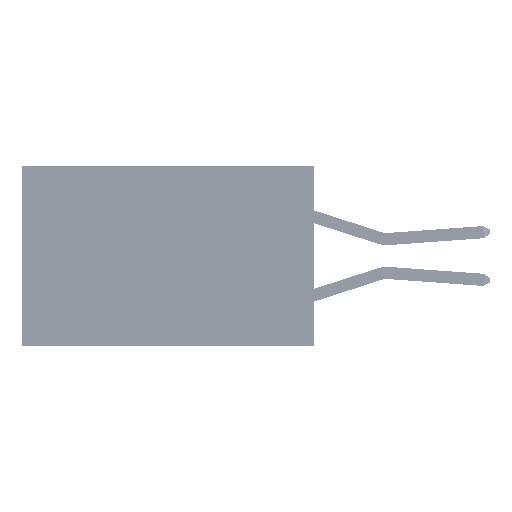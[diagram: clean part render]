
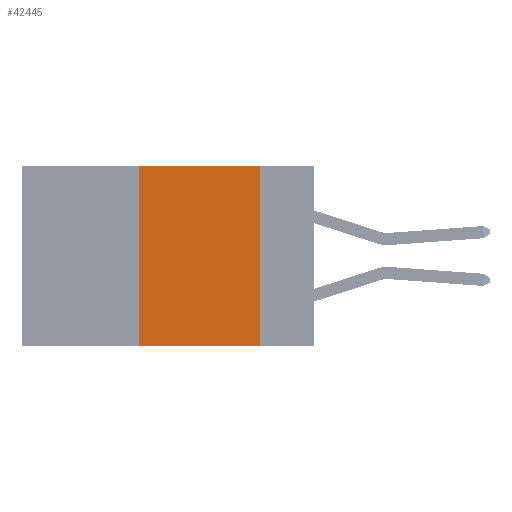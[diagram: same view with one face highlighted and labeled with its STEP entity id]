
A CAD part, left-side view. The second image highlights one B-rep face of the part: STEP entity #42445.
In plain terms, the highlighted planar face has unit normal (-1, 0, 0).
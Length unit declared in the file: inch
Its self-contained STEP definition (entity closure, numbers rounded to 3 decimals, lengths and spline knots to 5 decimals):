
#1733 = PLANE ( 'NONE',  #35816 ) ;
#5433 = EDGE_CURVE ( 'NONE', #27757, #46484, #41402, .T. ) ;
#5661 = DIRECTION ( 'NONE',  ( 1., 0., 0. ) ) ;
#5939 = CARTESIAN_POINT ( 'NONE',  ( 0., 0.6, 0. ) ) ;
#6447 = LINE ( 'NONE', #15994, #17030 ) ;
#6874 = ORIENTED_EDGE ( 'NONE', *, *, #20374, .T. ) ;
#7655 = FACE_OUTER_BOUND ( 'NONE', #9032, .T. ) ;
#9032 = EDGE_LOOP ( 'NONE', ( #36556, #16389, #25177, #6874 ) ) ;
#9548 = CARTESIAN_POINT ( 'NONE',  ( 0., 0.11, -0.37 ) ) ;
#11203 = DIRECTION ( 'NONE',  ( 0., 0., 1. ) ) ;
#13150 = LINE ( 'NONE', #33388, #15545 ) ;
#13716 = CARTESIAN_POINT ( 'NONE',  ( 0., 0.36, 0. ) ) ;
#13721 = DIRECTION ( 'NONE',  ( 0., 0., -1. ) ) ;
#15545 = VECTOR ( 'NONE', #25747, 39.37008 ) ;
#15994 = CARTESIAN_POINT ( 'NONE',  ( 0., 0.36, 0. ) ) ;
#16389 = ORIENTED_EDGE ( 'NONE', *, *, #5433, .F. ) ;
#16857 = VERTEX_POINT ( 'NONE', #9548 ) ;
#17030 = VECTOR ( 'NONE', #11203, 39.37008 ) ;
#20232 = DIRECTION ( 'NONE',  ( 0., -1., 0. ) ) ;
#20374 = EDGE_CURVE ( 'NONE', #37400, #16857, #13150, .T. ) ;
#22605 = EDGE_CURVE ( 'NONE', #37400, #27757, #6447, .T. ) ;
#25115 = CARTESIAN_POINT ( 'NONE',  ( 0., 0.11, 0. ) ) ;
#25177 = ORIENTED_EDGE ( 'NONE', *, *, #22605, .F. ) ;
#25747 = DIRECTION ( 'NONE',  ( 0., -1., 0. ) ) ;
#27757 = VERTEX_POINT ( 'NONE', #13716 ) ;
#28015 = CARTESIAN_POINT ( 'NONE',  ( 0., 0.6, 0. ) ) ;
#29764 = LINE ( 'NONE', #25115, #39119 ) ;
#31294 = EDGE_CURVE ( 'NONE', #46484, #16857, #29764, .T. ) ;
#33388 = CARTESIAN_POINT ( 'NONE',  ( 0., 0.6, -0.37 ) ) ;
#35057 = DIRECTION ( 'NONE',  ( 0., 0., -1. ) ) ;
#35816 = AXIS2_PLACEMENT_3D ( 'NONE', #28015, #5661, #35057 ) ;
#36556 = ORIENTED_EDGE ( 'NONE', *, *, #31294, .F. ) ;
#37274 = VECTOR ( 'NONE', #20232, 39.37008 ) ;
#37400 = VERTEX_POINT ( 'NONE', #44331 ) ;
#39119 = VECTOR ( 'NONE', #13721, 39.37008 ) ;
#39800 = CARTESIAN_POINT ( 'NONE',  ( 0., 0.11, 0. ) ) ;
#41402 = LINE ( 'NONE', #5939, #37274 ) ;
#42445 = ADVANCED_FACE ( 'NONE', ( #7655 ), #1733, .F. ) ;
#44331 = CARTESIAN_POINT ( 'NONE',  ( 0., 0.36, -0.37 ) ) ;
#46484 = VERTEX_POINT ( 'NONE', #39800 ) ;
